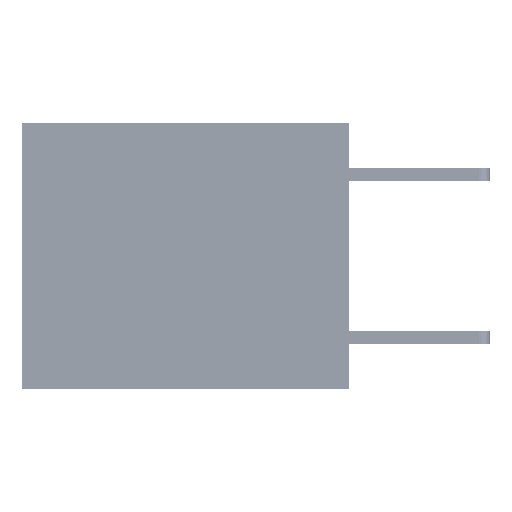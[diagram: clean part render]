
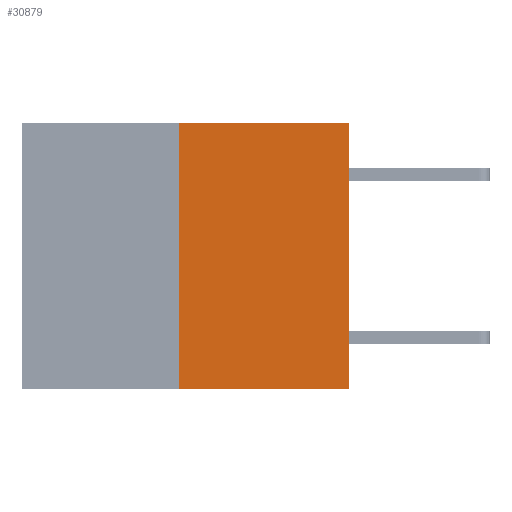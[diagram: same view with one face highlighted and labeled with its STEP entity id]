
A CAD part, left-side view. The second image highlights one B-rep face of the part: STEP entity #30879.
In plain terms, the highlighted planar face has unit normal (-1, 0, 0).
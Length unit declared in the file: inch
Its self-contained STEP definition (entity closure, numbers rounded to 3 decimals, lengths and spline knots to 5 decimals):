
#1004 = EDGE_CURVE ( 'NONE', #5896, #8334, #25052, .T. ) ;
#2466 = DIRECTION ( 'NONE',  ( 0., 0., 1. ) ) ;
#4267 = VECTOR ( 'NONE', #2466, 39.37008 ) ;
#5375 = CARTESIAN_POINT ( 'NONE',  ( 0., 0.6, 0. ) ) ;
#5546 = EDGE_LOOP ( 'NONE', ( #33388, #13557, #15717, #36147 ) ) ;
#5896 = VERTEX_POINT ( 'NONE', #5902 ) ;
#5902 = CARTESIAN_POINT ( 'NONE',  ( 0., 0.312, -0.49 ) ) ;
#7724 = DIRECTION ( 'NONE',  ( 0., 0., -1. ) ) ;
#8097 = PLANE ( 'NONE',  #12366 ) ;
#8334 = VERTEX_POINT ( 'NONE', #16124 ) ;
#8755 = DIRECTION ( 'NONE',  ( 0., -1., 0. ) ) ;
#9456 = LINE ( 'NONE', #5375, #31286 ) ;
#10506 = EDGE_CURVE ( 'NONE', #32547, #19369, #9456, .T. ) ;
#12366 = AXIS2_PLACEMENT_3D ( 'NONE', #30765, #32786, #7724 ) ;
#13557 = ORIENTED_EDGE ( 'NONE', *, *, #1004, .T. ) ;
#13952 = VECTOR ( 'NONE', #27030, 39.37008 ) ;
#15249 = VECTOR ( 'NONE', #21631, 39.37008 ) ;
#15717 = ORIENTED_EDGE ( 'NONE', *, *, #17918, .T. ) ;
#16124 = CARTESIAN_POINT ( 'NONE',  ( 0., 0., -0.49 ) ) ;
#17309 = CARTESIAN_POINT ( 'NONE',  ( 0., 0.312, 0. ) ) ;
#17918 = EDGE_CURVE ( 'NONE', #8334, #19369, #32273, .T. ) ;
#19369 = VERTEX_POINT ( 'NONE', #30551 ) ;
#21631 = DIRECTION ( 'NONE',  ( 0., -1., 0. ) ) ;
#24311 = LINE ( 'NONE', #35667, #4267 ) ;
#25052 = LINE ( 'NONE', #35879, #15249 ) ;
#27030 = DIRECTION ( 'NONE',  ( 0., 0., 1. ) ) ;
#27375 = FACE_OUTER_BOUND ( 'NONE', #5546, .T. ) ;
#30551 = CARTESIAN_POINT ( 'NONE',  ( 0., 0., 0. ) ) ;
#30765 = CARTESIAN_POINT ( 'NONE',  ( 0., 0.6, 0. ) ) ;
#30879 = ADVANCED_FACE ( 'NONE', ( #27375 ), #8097, .F. ) ;
#31286 = VECTOR ( 'NONE', #8755, 39.37008 ) ;
#32273 = LINE ( 'NONE', #34626, #13952 ) ;
#32547 = VERTEX_POINT ( 'NONE', #17309 ) ;
#32786 = DIRECTION ( 'NONE',  ( 1., 0., 0. ) ) ;
#33388 = ORIENTED_EDGE ( 'NONE', *, *, #34786, .F. ) ;
#34626 = CARTESIAN_POINT ( 'NONE',  ( 0., 0., 0. ) ) ;
#34786 = EDGE_CURVE ( 'NONE', #5896, #32547, #24311, .T. ) ;
#35667 = CARTESIAN_POINT ( 'NONE',  ( 0., 0.312, -0.49 ) ) ;
#35879 = CARTESIAN_POINT ( 'NONE',  ( 0., 0.6, -0.49 ) ) ;
#36147 = ORIENTED_EDGE ( 'NONE', *, *, #10506, .F. ) ;
